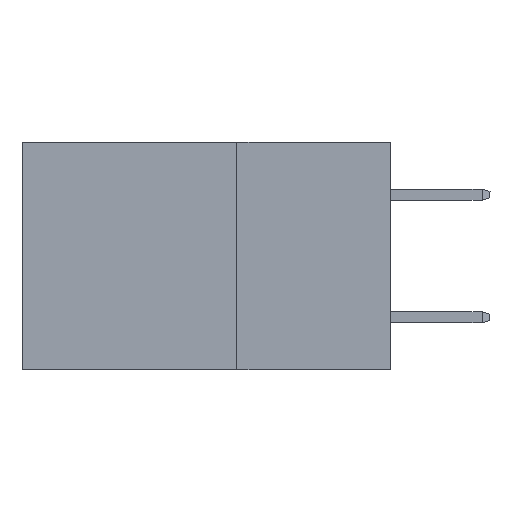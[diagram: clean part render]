
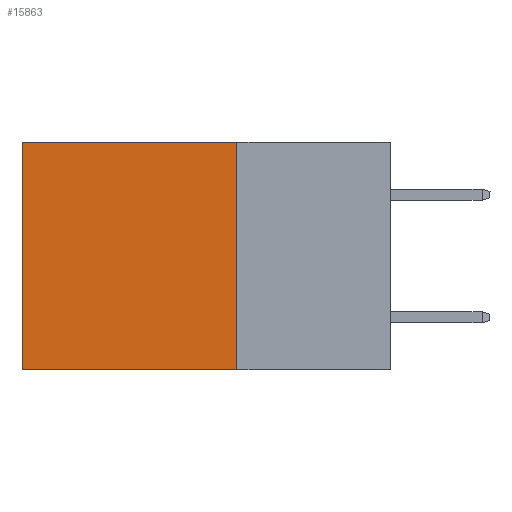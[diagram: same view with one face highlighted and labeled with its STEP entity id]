
A CAD part, left-side view. The second image highlights one B-rep face of the part: STEP entity #15863.
In plain terms, the highlighted planar face has unit normal (-1, 0, 0).
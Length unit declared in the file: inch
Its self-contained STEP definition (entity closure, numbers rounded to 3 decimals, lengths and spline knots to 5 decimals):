
#68 = CARTESIAN_POINT ( 'NONE',  ( 0.2875, 0.25, 0. ) ) ;
#358 = EDGE_CURVE ( 'NONE', #11833, #6464, #6385, .T. ) ;
#463 = CARTESIAN_POINT ( 'NONE',  ( 0.2875, 0.6, -0.37 ) ) ;
#996 = CARTESIAN_POINT ( 'NONE',  ( 0.2875, 0.25, 0. ) ) ;
#1208 = VECTOR ( 'NONE', #11487, 39.37008 ) ;
#1525 = CARTESIAN_POINT ( 'NONE',  ( 0.2875, 0.25, -0.37 ) ) ;
#2145 = CARTESIAN_POINT ( 'NONE',  ( 0.2875, 0.25, -0.37 ) ) ;
#2254 = CARTESIAN_POINT ( 'NONE',  ( 0.2875, 0.25, 0. ) ) ;
#2276 = DIRECTION ( 'NONE',  ( 0., 0., -1. ) ) ;
#2596 = ORIENTED_EDGE ( 'NONE', *, *, #5427, .F. ) ;
#2641 = EDGE_CURVE ( 'NONE', #13524, #6168, #10928, .T. ) ;
#4965 = DIRECTION ( 'NONE',  ( 0., 0., -1. ) ) ;
#5427 = EDGE_CURVE ( 'NONE', #11833, #13524, #8594, .T. ) ;
#5785 = ORIENTED_EDGE ( 'NONE', *, *, #10755, .T. ) ;
#6168 = VERTEX_POINT ( 'NONE', #463 ) ;
#6385 = LINE ( 'NONE', #68, #15600 ) ;
#6464 = VERTEX_POINT ( 'NONE', #15838 ) ;
#6853 = VECTOR ( 'NONE', #4965, 39.37008 ) ;
#8032 = EDGE_LOOP ( 'NONE', ( #5785, #10056, #2596, #12528 ) ) ;
#8088 = DIRECTION ( 'NONE',  ( 0., 1., 0. ) ) ;
#8181 = VECTOR ( 'NONE', #11234, 39.37008 ) ;
#8594 = LINE ( 'NONE', #12343, #8181 ) ;
#8700 = PLANE ( 'NONE',  #14799 ) ;
#9919 = DIRECTION ( 'NONE',  ( 1., 0., 0. ) ) ;
#10056 = ORIENTED_EDGE ( 'NONE', *, *, #2641, .F. ) ;
#10755 = EDGE_CURVE ( 'NONE', #6464, #6168, #13651, .T. ) ;
#10928 = LINE ( 'NONE', #2145, #1208 ) ;
#11214 = FACE_OUTER_BOUND ( 'NONE', #8032, .T. ) ;
#11234 = DIRECTION ( 'NONE',  ( 0., 0., -1. ) ) ;
#11487 = DIRECTION ( 'NONE',  ( 0., 1., 0. ) ) ;
#11833 = VERTEX_POINT ( 'NONE', #2254 ) ;
#12343 = CARTESIAN_POINT ( 'NONE',  ( 0.2875, 0.25, 0. ) ) ;
#12528 = ORIENTED_EDGE ( 'NONE', *, *, #358, .T. ) ;
#13524 = VERTEX_POINT ( 'NONE', #1525 ) ;
#13556 = CARTESIAN_POINT ( 'NONE',  ( 0.2875, 0.6, 0. ) ) ;
#13651 = LINE ( 'NONE', #13556, #6853 ) ;
#14799 = AXIS2_PLACEMENT_3D ( 'NONE', #996, #9919, #2276 ) ;
#15600 = VECTOR ( 'NONE', #8088, 39.37008 ) ;
#15838 = CARTESIAN_POINT ( 'NONE',  ( 0.2875, 0.6, 0. ) ) ;
#15863 = ADVANCED_FACE ( 'NONE', ( #11214 ), #8700, .F. ) ;
